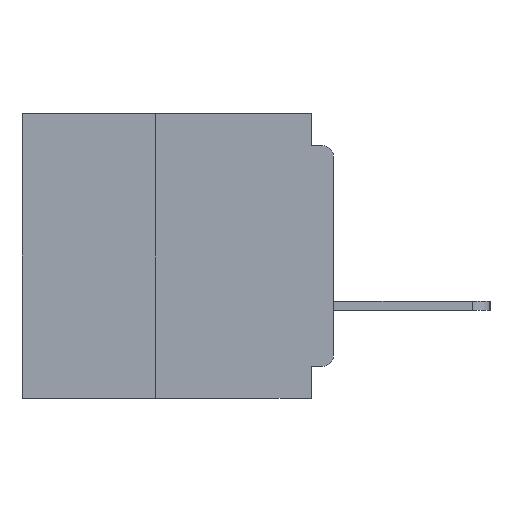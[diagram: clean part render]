
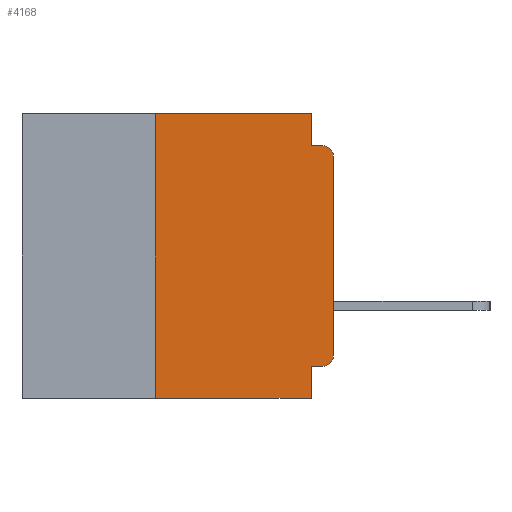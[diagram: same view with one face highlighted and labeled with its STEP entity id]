
A CAD part, left-side view. The second image highlights one B-rep face of the part: STEP entity #4168.
In plain terms, the highlighted planar face has unit normal (-1, 0, 0).
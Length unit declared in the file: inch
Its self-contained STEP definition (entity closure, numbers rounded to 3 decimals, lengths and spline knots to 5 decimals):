
#146 = CARTESIAN_POINT ( 'NONE',  ( 0., 0.031, 0. ) ) ;
#735 = VERTEX_POINT ( 'NONE', #4851 ) ;
#737 = EDGE_CURVE ( 'NONE', #735, #31165, #25064, .T. ) ;
#1115 = ORIENTED_EDGE ( 'NONE', *, *, #737, .F. ) ;
#1143 = DIRECTION ( 'NONE',  ( 0., -1., 0. ) ) ;
#1962 = VECTOR ( 'NONE', #27174, 39.37008 ) ;
#2185 = CARTESIAN_POINT ( 'NONE',  ( 0., 0.031, -0.4 ) ) ;
#2234 = ORIENTED_EDGE ( 'NONE', *, *, #10215, .F. ) ;
#2314 = VECTOR ( 'NONE', #10039, 39.37008 ) ;
#3030 = CIRCLE ( 'NONE', #16572, 0.015 ) ;
#4168 = ADVANCED_FACE ( 'NONE', ( #16955 ), #28760, .F. ) ;
#4577 = ORIENTED_EDGE ( 'NONE', *, *, #23473, .F. ) ;
#4851 = CARTESIAN_POINT ( 'NONE',  ( 0., 0.25, 0. ) ) ;
#4929 = CARTESIAN_POINT ( 'NONE',  ( 0., 0.437, 0. ) ) ;
#5236 = EDGE_CURVE ( 'NONE', #12856, #21963, #8300, .T. ) ;
#6069 = CARTESIAN_POINT ( 'NONE',  ( 0., 0.015, -0.355 ) ) ;
#6314 = VERTEX_POINT ( 'NONE', #15260 ) ;
#6636 = CARTESIAN_POINT ( 'NONE',  ( 0., 0.437, -0.4 ) ) ;
#7237 = EDGE_CURVE ( 'NONE', #21963, #18078, #3030, .T. ) ;
#7264 = VERTEX_POINT ( 'NONE', #11070 ) ;
#7437 = DIRECTION ( 'NONE',  ( 0., 0., 1. ) ) ;
#7448 = CARTESIAN_POINT ( 'NONE',  ( 0., 0., 0. ) ) ;
#7709 = DIRECTION ( 'NONE',  ( 0., 0., -1. ) ) ;
#8300 = LINE ( 'NONE', #7448, #15586 ) ;
#9188 = VERTEX_POINT ( 'NONE', #6069 ) ;
#9952 = EDGE_CURVE ( 'NONE', #6314, #24626, #26837, .T. ) ;
#10039 = DIRECTION ( 'NONE',  ( 0., -1., 0. ) ) ;
#10155 = VECTOR ( 'NONE', #15088, 39.37008 ) ;
#10215 = EDGE_CURVE ( 'NONE', #7264, #24626, #18300, .T. ) ;
#10960 = CARTESIAN_POINT ( 'NONE',  ( 0., 0.015, -0.06 ) ) ;
#11070 = CARTESIAN_POINT ( 'NONE',  ( 0., 0.031, -0.355 ) ) ;
#11126 = CARTESIAN_POINT ( 'NONE',  ( 0., 0., -0.06 ) ) ;
#11318 = DIRECTION ( 'NONE',  ( -1., 0., 0. ) ) ;
#11354 = VECTOR ( 'NONE', #1143, 39.37008 ) ;
#12856 = VERTEX_POINT ( 'NONE', #24099 ) ;
#12861 = AXIS2_PLACEMENT_3D ( 'NONE', #27764, #11318, #30424 ) ;
#13730 = DIRECTION ( 'NONE',  ( 0., 0., -1. ) ) ;
#15088 = DIRECTION ( 'NONE',  ( 0., 0., -1. ) ) ;
#15260 = CARTESIAN_POINT ( 'NONE',  ( 0., 0.25, -0.4 ) ) ;
#15586 = VECTOR ( 'NONE', #7437, 39.37008 ) ;
#15626 = ORIENTED_EDGE ( 'NONE', *, *, #25366, .F. ) ;
#16519 = CARTESIAN_POINT ( 'NONE',  ( 0., 0.015, -0.045 ) ) ;
#16546 = LINE ( 'NONE', #24328, #1962 ) ;
#16572 = AXIS2_PLACEMENT_3D ( 'NONE', #10960, #30074, #13730 ) ;
#16955 = FACE_OUTER_BOUND ( 'NONE', #20351, .T. ) ;
#17916 = AXIS2_PLACEMENT_3D ( 'NONE', #29111, #28412, #28378 ) ;
#18078 = VERTEX_POINT ( 'NONE', #16519 ) ;
#18300 = LINE ( 'NONE', #26870, #31838 ) ;
#19432 = LINE ( 'NONE', #20975, #31250 ) ;
#20351 = EDGE_LOOP ( 'NONE', ( #21041, #32052, #15626, #34683, #1115, #4577, #29467, #2234, #32513, #20679 ) ) ;
#20679 = ORIENTED_EDGE ( 'NONE', *, *, #26654, .T. ) ;
#20975 = CARTESIAN_POINT ( 'NONE',  ( 0., 0., -0.355 ) ) ;
#21041 = ORIENTED_EDGE ( 'NONE', *, *, #5236, .T. ) ;
#21963 = VERTEX_POINT ( 'NONE', #11126 ) ;
#23021 = EDGE_CURVE ( 'NONE', #9188, #7264, #19432, .T. ) ;
#23220 = VECTOR ( 'NONE', #33880, 39.37008 ) ;
#23473 = EDGE_CURVE ( 'NONE', #6314, #735, #31217, .T. ) ;
#24099 = CARTESIAN_POINT ( 'NONE',  ( 0., 0., -0.34 ) ) ;
#24220 = CIRCLE ( 'NONE', #12861, 0.015 ) ;
#24328 = CARTESIAN_POINT ( 'NONE',  ( 0., 0., -0.045 ) ) ;
#24626 = VERTEX_POINT ( 'NONE', #2185 ) ;
#24758 = LINE ( 'NONE', #28723, #10155 ) ;
#25064 = LINE ( 'NONE', #4929, #2314 ) ;
#25366 = EDGE_CURVE ( 'NONE', #27391, #18078, #16546, .T. ) ;
#25571 = CARTESIAN_POINT ( 'NONE',  ( 0., 0.031, -0.045 ) ) ;
#26654 = EDGE_CURVE ( 'NONE', #9188, #12856, #24220, .T. ) ;
#26837 = LINE ( 'NONE', #6636, #11354 ) ;
#26870 = CARTESIAN_POINT ( 'NONE',  ( 0., 0.031, -0.4 ) ) ;
#27174 = DIRECTION ( 'NONE',  ( 0., -1., 0. ) ) ;
#27391 = VERTEX_POINT ( 'NONE', #25571 ) ;
#27764 = CARTESIAN_POINT ( 'NONE',  ( 0., 0.015, -0.34 ) ) ;
#28378 = DIRECTION ( 'NONE',  ( 0., 0., -1. ) ) ;
#28412 = DIRECTION ( 'NONE',  ( 1., 0., 0. ) ) ;
#28723 = CARTESIAN_POINT ( 'NONE',  ( 0., 0.031, 0. ) ) ;
#28760 = PLANE ( 'NONE',  #17916 ) ;
#29111 = CARTESIAN_POINT ( 'NONE',  ( 0., 0.437, 0. ) ) ;
#29467 = ORIENTED_EDGE ( 'NONE', *, *, #9952, .T. ) ;
#30074 = DIRECTION ( 'NONE',  ( -1., 0., 0. ) ) ;
#30424 = DIRECTION ( 'NONE',  ( 0., 0., -1. ) ) ;
#30838 = EDGE_CURVE ( 'NONE', #31165, #27391, #24758, .T. ) ;
#31165 = VERTEX_POINT ( 'NONE', #146 ) ;
#31175 = CARTESIAN_POINT ( 'NONE',  ( 0., 0.25, -0.4 ) ) ;
#31217 = LINE ( 'NONE', #31175, #23220 ) ;
#31250 = VECTOR ( 'NONE', #34514, 39.37008 ) ;
#31838 = VECTOR ( 'NONE', #7709, 39.37008 ) ;
#32052 = ORIENTED_EDGE ( 'NONE', *, *, #7237, .T. ) ;
#32513 = ORIENTED_EDGE ( 'NONE', *, *, #23021, .F. ) ;
#33880 = DIRECTION ( 'NONE',  ( 0., 0., 1. ) ) ;
#34514 = DIRECTION ( 'NONE',  ( 0., 1., 0. ) ) ;
#34683 = ORIENTED_EDGE ( 'NONE', *, *, #30838, .F. ) ;
